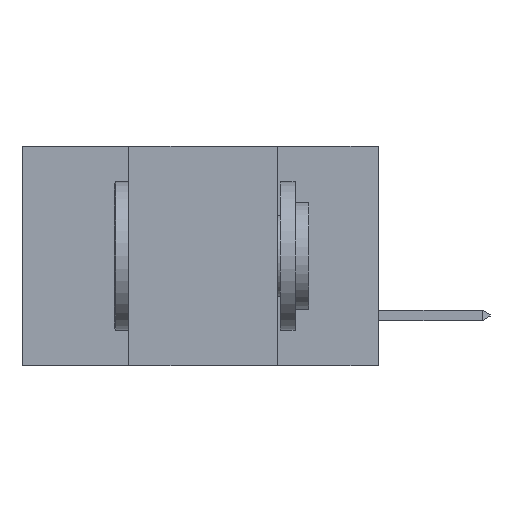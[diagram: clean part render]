
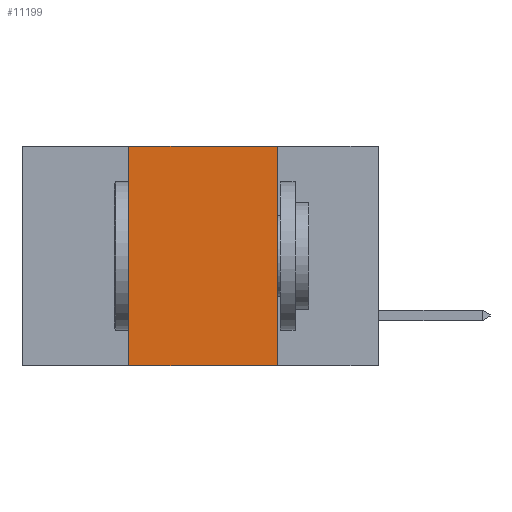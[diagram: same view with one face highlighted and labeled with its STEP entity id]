
A CAD part, left-side view. The second image highlights one B-rep face of the part: STEP entity #11199.
In plain terms, the highlighted planar face has unit normal (-1, 0, 0).
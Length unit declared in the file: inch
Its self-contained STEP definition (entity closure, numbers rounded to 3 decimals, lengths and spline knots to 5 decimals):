
#638 = DIRECTION ( 'NONE',  ( 0., 0., 1. ) ) ;
#668 = CARTESIAN_POINT ( 'NONE',  ( 0., 0.17, 0. ) ) ;
#804 = CARTESIAN_POINT ( 'NONE',  ( 0., 0.42, -0.37 ) ) ;
#880 = CARTESIAN_POINT ( 'NONE',  ( 0., 0.6, 0. ) ) ;
#1447 = CARTESIAN_POINT ( 'NONE',  ( 0., 0.17, 0. ) ) ;
#1468 = DIRECTION ( 'NONE',  ( 0., 0., -1. ) ) ;
#1942 = DIRECTION ( 'NONE',  ( 1., 0., 0. ) ) ;
#2092 = CARTESIAN_POINT ( 'NONE',  ( 0., 0.42, 0. ) ) ;
#2404 = LINE ( 'NONE', #11267, #10147 ) ;
#2702 = ORIENTED_EDGE ( 'NONE', *, *, #4170, .F. ) ;
#4154 = VERTEX_POINT ( 'NONE', #12264 ) ;
#4170 = EDGE_CURVE ( 'NONE', #10510, #5305, #5723, .T. ) ;
#5175 = EDGE_CURVE ( 'NONE', #10510, #4154, #11765, .T. ) ;
#5305 = VERTEX_POINT ( 'NONE', #2092 ) ;
#5723 = LINE ( 'NONE', #9176, #10723 ) ;
#5924 = FACE_OUTER_BOUND ( 'NONE', #10371, .T. ) ;
#5937 = EDGE_CURVE ( 'NONE', #5305, #10426, #2404, .T. ) ;
#6300 = CARTESIAN_POINT ( 'NONE',  ( 0., 0.6, -0.37 ) ) ;
#6457 = VECTOR ( 'NONE', #9445, 39.37008 ) ;
#6985 = PLANE ( 'NONE',  #10733 ) ;
#7691 = EDGE_CURVE ( 'NONE', #10426, #4154, #10404, .T. ) ;
#9020 = DIRECTION ( 'NONE',  ( 0., 0., -1. ) ) ;
#9176 = CARTESIAN_POINT ( 'NONE',  ( 0., 0.42, 0. ) ) ;
#9445 = DIRECTION ( 'NONE',  ( 0., -1., 0. ) ) ;
#9678 = ORIENTED_EDGE ( 'NONE', *, *, #5175, .T. ) ;
#10098 = VECTOR ( 'NONE', #1468, 39.37008 ) ;
#10120 = ORIENTED_EDGE ( 'NONE', *, *, #5937, .F. ) ;
#10147 = VECTOR ( 'NONE', #12646, 39.37008 ) ;
#10371 = EDGE_LOOP ( 'NONE', ( #11498, #10120, #2702, #9678 ) ) ;
#10404 = LINE ( 'NONE', #1447, #10098 ) ;
#10426 = VERTEX_POINT ( 'NONE', #668 ) ;
#10510 = VERTEX_POINT ( 'NONE', #804 ) ;
#10723 = VECTOR ( 'NONE', #638, 39.37008 ) ;
#10733 = AXIS2_PLACEMENT_3D ( 'NONE', #880, #1942, #9020 ) ;
#11199 = ADVANCED_FACE ( 'NONE', ( #5924 ), #6985, .F. ) ;
#11267 = CARTESIAN_POINT ( 'NONE',  ( 0., 0.6, 0. ) ) ;
#11498 = ORIENTED_EDGE ( 'NONE', *, *, #7691, .F. ) ;
#11765 = LINE ( 'NONE', #6300, #6457 ) ;
#12264 = CARTESIAN_POINT ( 'NONE',  ( 0., 0.17, -0.37 ) ) ;
#12646 = DIRECTION ( 'NONE',  ( 0., -1., 0. ) ) ;
